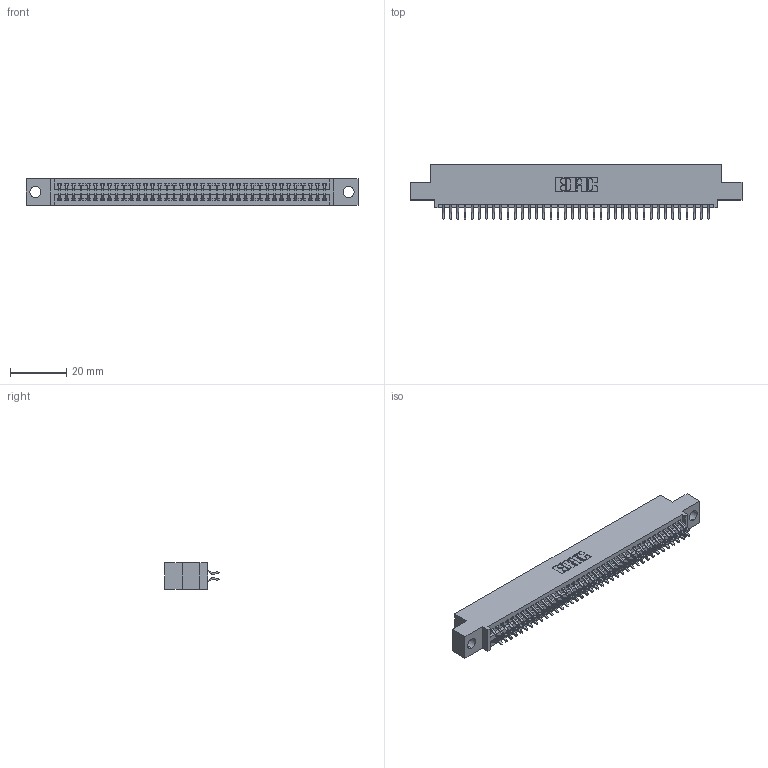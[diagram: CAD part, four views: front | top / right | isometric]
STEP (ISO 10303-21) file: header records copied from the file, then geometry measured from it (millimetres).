
FILE_DESCRIPTION (( 'STEP AP203' ), '1' );
FILE_NAME ('395-076-556-504.STEP', '2021-06-17T06:13:16', ( '' ), ( '' ), 'SwSTEP 2.0', 'SolidWorks 2020', '' );
FILE_SCHEMA (( 'CONFIG_CONTROL_DESIGN' ));
Length unit declared in the file: inch
Products named in the file (3): 395-076-556-504; 345 Part_0.110 Offset - 0.156 Dia-TI; 345-292-001_556 Tail
Assembly tree (77 placements, depth 2):
  395-076-556-504
    345 Part_0.110 Offset - 0.156 Dia-TI
    345-292-001_556 Tail  x76
Bounding box: 117.73 x 19.24 x 9.4 mm (x, y, z)
Volume: 11216.9 mm3; surface area: 16380.8 mm2
Topology: 77 solids, 77 shells, 4400 faces, 13081 edges, 8618 vertices
Faces by surface type: plane 2910, cylinder 1490
Entity records: 31125 total; most frequent: CARTESIAN_POINT 5242, ORIENTED_EDGE 5162, DIRECTION 4613, EDGE_CURVE 2581, VECTOR 2289, LINE 2289, VERTEX_POINT 1718, AXIS2_PLACEMENT_3D 1162
